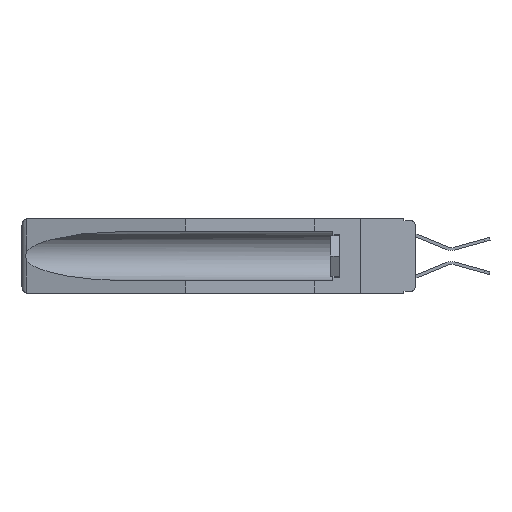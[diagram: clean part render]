
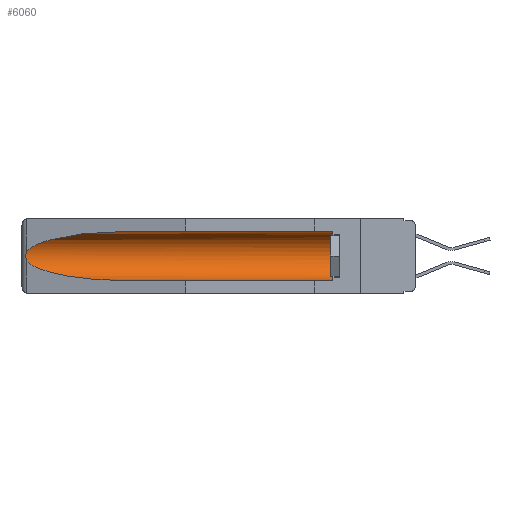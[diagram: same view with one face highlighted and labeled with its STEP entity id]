
A CAD part, left-side view. The second image highlights one B-rep face of the part: STEP entity #6060.
In plain terms, the highlighted cylindrical face has radius 2.857 mm (diameter 5.715 mm), a partial arc.
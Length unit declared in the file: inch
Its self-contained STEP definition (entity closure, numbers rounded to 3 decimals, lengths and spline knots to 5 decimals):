
#1077 = AXIS2_PLACEMENT_3D ( 'NONE', #4362, #8674, #13088 ) ;
#1377 = VERTEX_POINT ( 'NONE', #9902 ) ;
#1392 = VECTOR ( 'NONE', #2165, 39.37008 ) ;
#1921 = AXIS2_PLACEMENT_3D ( 'NONE', #2609, #12652, #3932 ) ;
#2165 = DIRECTION ( 'NONE',  ( 0., 1., 0. ) ) ;
#2341 = ORIENTED_EDGE ( 'NONE', *, *, #5478, .T. ) ;
#2609 = CARTESIAN_POINT ( 'NONE',  ( 0.155, -0.30754, -0.1715 ) ) ;
#2753 = CARTESIAN_POINT ( 'NONE',  ( 0.155, -0.30754, -0.284 ) ) ;
#2836 = ORIENTED_EDGE ( 'NONE', *, *, #10565, .T. ) ;
#2981 = ORIENTED_EDGE ( 'NONE', *, *, #16922, .T. ) ;
#3321 = EDGE_LOOP ( 'NONE', ( #2341, #2836, #2981, #12575, #15775, #8153 ) ) ;
#3740 = VERTEX_POINT ( 'NONE', #18476 ) ;
#3932 = DIRECTION ( 'NONE',  ( 0., 0., 1. ) ) ;
#4362 = CARTESIAN_POINT ( 'NONE',  ( 0.155, 0.126, -0.1715 ) ) ;
#4774 = CARTESIAN_POINT ( 'NONE',  ( 0.2673, 1.53269, -0.17917 ) ) ;
#5229 = FACE_OUTER_BOUND ( 'NONE', #3321, .T. ) ;
#5478 = EDGE_CURVE ( 'NONE', #17205, #8117, #14395, .T. ) ;
#5577 = CARTESIAN_POINT ( 'NONE',  ( 0.155, 1.07973, -0.059 ) ) ;
#6060 = ADVANCED_FACE ( 'NONE', ( #5229 ), #14034, .F. ) ;
#6200 = CARTESIAN_POINT ( 'NONE',  ( 0.26654, 1.53092, -0.15636 ) ) ;
#6230 = CARTESIAN_POINT ( 'NONE',  ( 0.25451, 1.48313, -0.09465 ) ) ;
#6860 = DIRECTION ( 'NONE',  ( 0., 1., 0. ) ) ;
#7050 = CIRCLE ( 'NONE', #1077, 0.1125 ) ;
#7090 = CARTESIAN_POINT ( 'NONE',  ( 0.26537, 1.52718, -0.19328 ) ) ;
#7229 = EDGE_CURVE ( 'NONE', #1377, #10248, #7050, .T. ) ;
#8093 = CARTESIAN_POINT ( 'NONE',  ( 0.21114, 1.30732, -0.059 ) ) ;
#8117 = VERTEX_POINT ( 'NONE', #14955 ) ;
#8153 = ORIENTED_EDGE ( 'NONE', *, *, #9144, .T. ) ;
#8169 = LINE ( 'NONE', #2753, #17268 ) ;
#8674 = DIRECTION ( 'NONE',  ( 0., -1., 0. ) ) ;
#8896 = EDGE_CURVE ( 'NONE', #1377, #3740, #8169, .T. ) ;
#9144 = EDGE_CURVE ( 'NONE', #10248, #17205, #14982, .T. ) ;
#9250 =( BOUNDED_CURVE ( )  B_SPLINE_CURVE ( 3, ( #7090, #10096, #11414, #18420 ),
 .UNSPECIFIED., .F., .T. ) 
 B_SPLINE_CURVE_WITH_KNOTS ( ( 4, 4 ),
 ( 0.1948, 1.5708 ),
 .UNSPECIFIED. ) 
 CURVE ( )  GEOMETRIC_REPRESENTATION_ITEM ( )  RATIONAL_B_SPLINE_CURVE ( ( 1., 0.848, 0.848, 1. ) ) 
 REPRESENTATION_ITEM ( '' )  );
#9902 = CARTESIAN_POINT ( 'NONE',  ( 0.155, 0.126, -0.284 ) ) ;
#10096 = CARTESIAN_POINT ( 'NONE',  ( 0.25451, 1.48313, -0.24835 ) ) ;
#10248 = VERTEX_POINT ( 'NONE', #18206 ) ;
#10440 = B_SPLINE_CURVE_WITH_KNOTS ( 'NONE', 3,
 ( #10789, #14894, #6200, #11926, #16492, #17641, #4774, #10511, #13949, #12759 ),
 .UNSPECIFIED., .F., .F.,
 ( 4, 2, 2, 2, 4 ),
 ( 0., 0.00029, 0.00058, 0.00087, 0.00117 ),
 .UNSPECIFIED. ) ;
#10511 = CARTESIAN_POINT ( 'NONE',  ( 0.26655, 1.53094, -0.18657 ) ) ;
#10565 = EDGE_CURVE ( 'NONE', #8117, #16533, #10440, .T. ) ;
#10789 = CARTESIAN_POINT ( 'NONE',  ( 0.26537, 1.52718, -0.14972 ) ) ;
#11337 = CARTESIAN_POINT ( 'NONE',  ( 0.26537, 1.52718, -0.19328 ) ) ;
#11414 = CARTESIAN_POINT ( 'NONE',  ( 0.21114, 1.30732, -0.284 ) ) ;
#11926 = CARTESIAN_POINT ( 'NONE',  ( 0.2673, 1.5327, -0.16383 ) ) ;
#12322 = CARTESIAN_POINT ( 'NONE',  ( 0.155, 1.07973, -0.059 ) ) ;
#12575 = ORIENTED_EDGE ( 'NONE', *, *, #8896, .F. ) ;
#12652 = DIRECTION ( 'NONE',  ( 0., 1., 0. ) ) ;
#12759 = CARTESIAN_POINT ( 'NONE',  ( 0.26537, 1.52718, -0.19328 ) ) ;
#13088 = DIRECTION ( 'NONE',  ( 0., 0., 1. ) ) ;
#13334 = CARTESIAN_POINT ( 'NONE',  ( 0.155, -0.30754, -0.059 ) ) ;
#13949 = CARTESIAN_POINT ( 'NONE',  ( 0.26597, 1.5296, -0.19026 ) ) ;
#14034 = CYLINDRICAL_SURFACE ( 'NONE', #1921, 0.1125 ) ;
#14395 =( BOUNDED_CURVE ( )  B_SPLINE_CURVE ( 3, ( #12322, #8093, #6230, #15189 ),
 .UNSPECIFIED., .F., .T. ) 
 B_SPLINE_CURVE_WITH_KNOTS ( ( 4, 4 ),
 ( 4.71239, 6.08839 ),
 .UNSPECIFIED. ) 
 CURVE ( )  GEOMETRIC_REPRESENTATION_ITEM ( )  RATIONAL_B_SPLINE_CURVE ( ( 1., 0.848, 0.848, 1. ) ) 
 REPRESENTATION_ITEM ( '' )  );
#14894 = CARTESIAN_POINT ( 'NONE',  ( 0.26597, 1.52961, -0.15275 ) ) ;
#14955 = CARTESIAN_POINT ( 'NONE',  ( 0.26537, 1.52718, -0.14972 ) ) ;
#14982 = LINE ( 'NONE', #13334, #1392 ) ;
#15189 = CARTESIAN_POINT ( 'NONE',  ( 0.26537, 1.52718, -0.14972 ) ) ;
#15775 = ORIENTED_EDGE ( 'NONE', *, *, #7229, .T. ) ;
#16492 = CARTESIAN_POINT ( 'NONE',  ( 0.2675, 1.53308, -0.16763 ) ) ;
#16533 = VERTEX_POINT ( 'NONE', #11337 ) ;
#16922 = EDGE_CURVE ( 'NONE', #16533, #3740, #9250, .T. ) ;
#17205 = VERTEX_POINT ( 'NONE', #5577 ) ;
#17268 = VECTOR ( 'NONE', #6860, 39.37008 ) ;
#17641 = CARTESIAN_POINT ( 'NONE',  ( 0.2675, 1.53308, -0.17534 ) ) ;
#18206 = CARTESIAN_POINT ( 'NONE',  ( 0.155, 0.126, -0.059 ) ) ;
#18420 = CARTESIAN_POINT ( 'NONE',  ( 0.155, 1.07973, -0.284 ) ) ;
#18476 = CARTESIAN_POINT ( 'NONE',  ( 0.155, 1.07973, -0.284 ) ) ;
